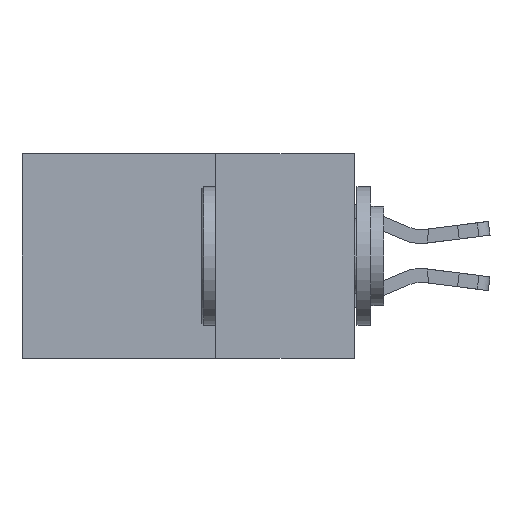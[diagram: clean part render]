
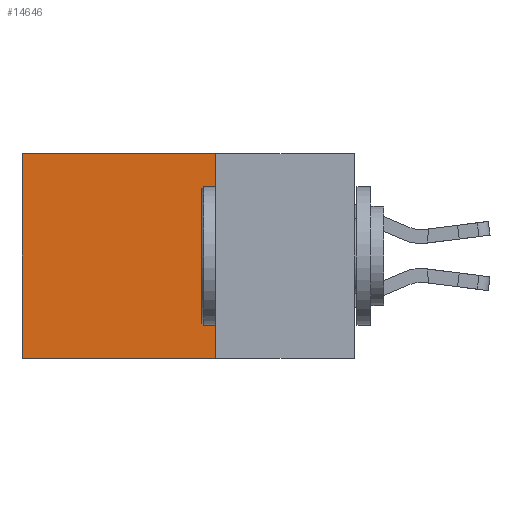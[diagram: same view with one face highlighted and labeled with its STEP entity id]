
A CAD part, left-side view. The second image highlights one B-rep face of the part: STEP entity #14646.
In plain terms, the highlighted planar face has unit normal (-1, 0, 0).
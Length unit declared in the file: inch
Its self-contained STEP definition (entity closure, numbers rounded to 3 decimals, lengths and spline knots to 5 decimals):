
#471 = CARTESIAN_POINT ( 'NONE',  ( 0.298, 0.25, -0.37 ) ) ;
#1770 = FACE_OUTER_BOUND ( 'NONE', #2225, .T. ) ;
#2059 = CARTESIAN_POINT ( 'NONE',  ( 0.298, 0.6, 0. ) ) ;
#2225 = EDGE_LOOP ( 'NONE', ( #11398, #12632, #21780, #6344 ) ) ;
#2759 = LINE ( 'NONE', #17262, #16585 ) ;
#2787 = DIRECTION ( 'NONE',  ( 0., 0., -1. ) ) ;
#3653 = DIRECTION ( 'NONE',  ( 0., 1., 0. ) ) ;
#4500 = EDGE_CURVE ( 'NONE', #17034, #16293, #5848, .T. ) ;
#5599 = EDGE_CURVE ( 'NONE', #5688, #18834, #13993, .T. ) ;
#5688 = VERTEX_POINT ( 'NONE', #471 ) ;
#5848 = LINE ( 'NONE', #10793, #7855 ) ;
#6344 = ORIENTED_EDGE ( 'NONE', *, *, #4500, .T. ) ;
#6549 = DIRECTION ( 'NONE',  ( 0., 0., -1. ) ) ;
#7855 = VECTOR ( 'NONE', #3653, 39.37008 ) ;
#8470 = LINE ( 'NONE', #22750, #16280 ) ;
#9248 = EDGE_CURVE ( 'NONE', #16293, #18834, #8470, .T. ) ;
#10793 = CARTESIAN_POINT ( 'NONE',  ( 0.298, 0.25, 0. ) ) ;
#11398 = ORIENTED_EDGE ( 'NONE', *, *, #9248, .T. ) ;
#11868 = CARTESIAN_POINT ( 'NONE',  ( 0.298, 0.25, 0. ) ) ;
#12632 = ORIENTED_EDGE ( 'NONE', *, *, #5599, .F. ) ;
#13346 = AXIS2_PLACEMENT_3D ( 'NONE', #11868, #13666, #2787 ) ;
#13429 = CARTESIAN_POINT ( 'NONE',  ( 0.298, 0.25, -0.37 ) ) ;
#13666 = DIRECTION ( 'NONE',  ( 1., 0., 0. ) ) ;
#13993 = LINE ( 'NONE', #13429, #22795 ) ;
#14646 = ADVANCED_FACE ( 'NONE', ( #1770 ), #22430, .F. ) ;
#16280 = VECTOR ( 'NONE', #21072, 39.37008 ) ;
#16293 = VERTEX_POINT ( 'NONE', #2059 ) ;
#16585 = VECTOR ( 'NONE', #6549, 39.37008 ) ;
#16943 = CARTESIAN_POINT ( 'NONE',  ( 0.298, 0.25, 0. ) ) ;
#17034 = VERTEX_POINT ( 'NONE', #16943 ) ;
#17262 = CARTESIAN_POINT ( 'NONE',  ( 0.298, 0.25, 0. ) ) ;
#18701 = CARTESIAN_POINT ( 'NONE',  ( 0.298, 0.6, -0.37 ) ) ;
#18834 = VERTEX_POINT ( 'NONE', #18701 ) ;
#20187 = EDGE_CURVE ( 'NONE', #17034, #5688, #2759, .T. ) ;
#21072 = DIRECTION ( 'NONE',  ( 0., 0., -1. ) ) ;
#21780 = ORIENTED_EDGE ( 'NONE', *, *, #20187, .F. ) ;
#22060 = DIRECTION ( 'NONE',  ( 0., 1., 0. ) ) ;
#22430 = PLANE ( 'NONE',  #13346 ) ;
#22750 = CARTESIAN_POINT ( 'NONE',  ( 0.298, 0.6, 0. ) ) ;
#22795 = VECTOR ( 'NONE', #22060, 39.37008 ) ;
